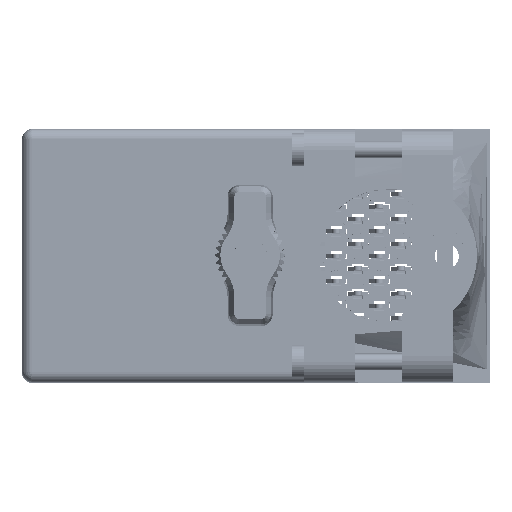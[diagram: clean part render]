
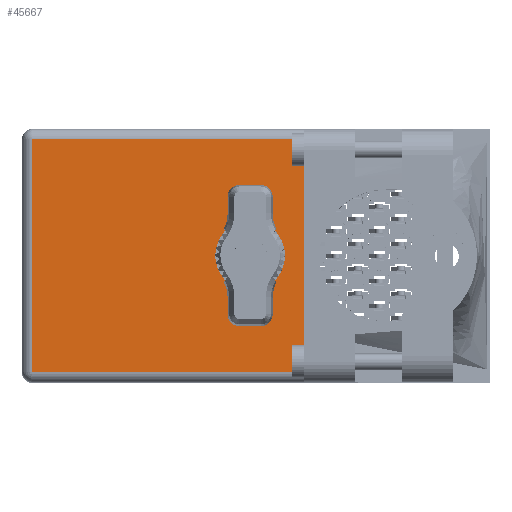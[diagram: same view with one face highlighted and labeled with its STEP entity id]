
A CAD part, top view. The second image highlights one B-rep face of the part: STEP entity #45667.
In plain terms, the highlighted face is planar.
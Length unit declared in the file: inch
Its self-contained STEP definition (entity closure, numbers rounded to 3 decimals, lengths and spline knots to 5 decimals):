
#563 = CARTESIAN_POINT ( 'NONE',  ( -1.3155, 1.93, -0.703 ) ) ;
#678 = ORIENTED_EDGE ( 'NONE', *, *, #26397, .T. ) ;
#2514 = VERTEX_POINT ( 'NONE', #80409 ) ;
#5912 = ORIENTED_EDGE ( 'NONE', *, *, #95374, .F. ) ;
#6459 = CARTESIAN_POINT ( 'NONE',  ( 0., 1.93, -0.17 ) ) ;
#9672 = LINE ( 'NONE', #101039, #72297 ) ;
#13199 = DIRECTION ( 'NONE',  ( 0., 1., 0. ) ) ;
#14090 = CIRCLE ( 'NONE', #49636, 0.17 ) ;
#18101 = VECTOR ( 'NONE', #20046, 39.37008 ) ;
#18230 = VECTOR ( 'NONE', #105249, 39.37008 ) ;
#20046 = DIRECTION ( 'NONE',  ( 1., 0., 0. ) ) ;
#22136 = DIRECTION ( 'NONE',  ( 0., 0., 1. ) ) ;
#23351 = LINE ( 'NONE', #48913, #18230 ) ;
#23357 = VERTEX_POINT ( 'NONE', #563 ) ;
#24147 = EDGE_CURVE ( 'NONE', #23357, #2514, #9672, .T. ) ;
#25440 = AXIS2_PLACEMENT_3D ( 'NONE', #43024, #34441, #100398 ) ;
#25984 = VERTEX_POINT ( 'NONE', #86287 ) ;
#26397 = EDGE_CURVE ( 'NONE', #56697, #23357, #102386, .T. ) ;
#26608 = DIRECTION ( 'NONE',  ( 0., 0., 1. ) ) ;
#26620 = CARTESIAN_POINT ( 'NONE',  ( -1.3775, 1.93, -0.703 ) ) ;
#28460 = VECTOR ( 'NONE', #83668, 39.37008 ) ;
#29287 = CARTESIAN_POINT ( 'NONE',  ( 0.3275, 1.93, 0.703 ) ) ;
#31080 = FACE_BOUND ( 'NONE', #103650, .T. ) ;
#31158 = VERTEX_POINT ( 'NONE', #6459 ) ;
#34441 = DIRECTION ( 'NONE',  ( 0., 1., 0. ) ) ;
#34677 = LINE ( 'NONE', #29287, #18101 ) ;
#43024 = CARTESIAN_POINT ( 'NONE',  ( -1.3775, 1.93, -0.765 ) ) ;
#45440 = EDGE_CURVE ( 'NONE', #31158, #60900, #105188, .T. ) ;
#45667 = ADVANCED_FACE ( 'NONE', ( #68007, #31080 ), #58715, .T. ) ;
#48913 = CARTESIAN_POINT ( 'NONE',  ( 0.3275, 1.93, -0.765 ) ) ;
#49636 = AXIS2_PLACEMENT_3D ( 'NONE', #75471, #76201, #26608 ) ;
#52586 = DIRECTION ( 'NONE',  ( 0., 0., 1. ) ) ;
#52602 = EDGE_LOOP ( 'NONE', ( #92591, #71976, #97911, #678 ) ) ;
#56697 = VERTEX_POINT ( 'NONE', #56963 ) ;
#56963 = CARTESIAN_POINT ( 'NONE',  ( 0.3275, 1.93, -0.703 ) ) ;
#58715 = PLANE ( 'NONE',  #25440 ) ;
#60900 = VERTEX_POINT ( 'NONE', #91096 ) ;
#62827 = CARTESIAN_POINT ( 'NONE',  ( 0., 1.93, 0. ) ) ;
#65172 = EDGE_CURVE ( 'NONE', #2514, #25984, #34677, .T. ) ;
#66360 = AXIS2_PLACEMENT_3D ( 'NONE', #62827, #13199, #22136 ) ;
#68007 = FACE_OUTER_BOUND ( 'NONE', #52602, .T. ) ;
#71976 = ORIENTED_EDGE ( 'NONE', *, *, #65172, .T. ) ;
#72297 = VECTOR ( 'NONE', #52586, 39.37008 ) ;
#74428 = ORIENTED_EDGE ( 'NONE', *, *, #45440, .F. ) ;
#75471 = CARTESIAN_POINT ( 'NONE',  ( 0., 1.93, 0. ) ) ;
#76201 = DIRECTION ( 'NONE',  ( 0., 1., 0. ) ) ;
#76615 = EDGE_CURVE ( 'NONE', #56697, #25984, #23351, .T. ) ;
#80409 = CARTESIAN_POINT ( 'NONE',  ( -1.3155, 1.93, 0.703 ) ) ;
#83668 = DIRECTION ( 'NONE',  ( -1., 0., 0. ) ) ;
#86287 = CARTESIAN_POINT ( 'NONE',  ( 0.3275, 1.93, 0.703 ) ) ;
#91096 = CARTESIAN_POINT ( 'NONE',  ( 0., 1.93, 0.17 ) ) ;
#92591 = ORIENTED_EDGE ( 'NONE', *, *, #24147, .T. ) ;
#95374 = EDGE_CURVE ( 'NONE', #60900, #31158, #14090, .T. ) ;
#97911 = ORIENTED_EDGE ( 'NONE', *, *, #76615, .F. ) ;
#100398 = DIRECTION ( 'NONE',  ( -1., 0., 0. ) ) ;
#101039 = CARTESIAN_POINT ( 'NONE',  ( -1.3155, 1.93, -0.765 ) ) ;
#102386 = LINE ( 'NONE', #26620, #28460 ) ;
#103650 = EDGE_LOOP ( 'NONE', ( #5912, #74428 ) ) ;
#105188 = CIRCLE ( 'NONE', #66360, 0.17 ) ;
#105249 = DIRECTION ( 'NONE',  ( 0., 0., 1. ) ) ;
